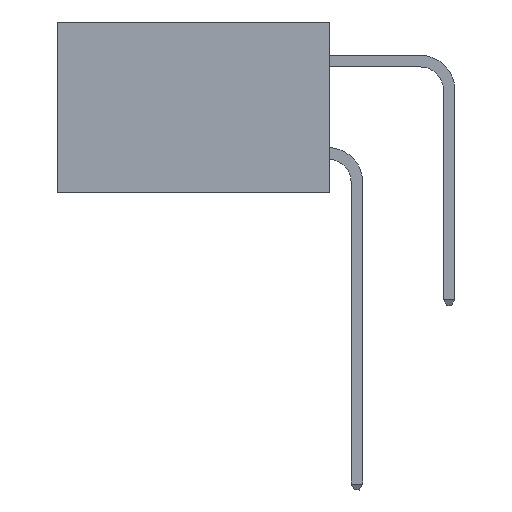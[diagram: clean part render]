
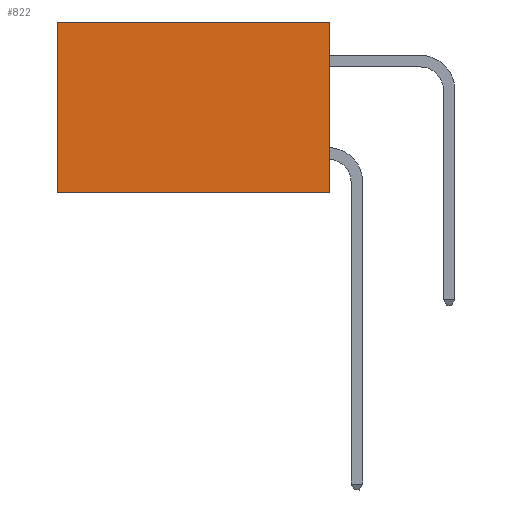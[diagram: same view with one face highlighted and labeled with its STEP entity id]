
A CAD part, left-side view. The second image highlights one B-rep face of the part: STEP entity #822.
In plain terms, the highlighted planar face has unit normal (-1, 0, 0).
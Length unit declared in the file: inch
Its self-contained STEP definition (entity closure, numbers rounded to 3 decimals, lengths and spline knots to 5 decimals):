
#822 = ADVANCED_FACE ( 'NONE', ( #1103 ), #14739, .F. ) ;
#1103 = FACE_OUTER_BOUND ( 'NONE', #1572, .T. ) ;
#1252 = VECTOR ( 'NONE', #8957, 39.37008 ) ;
#1416 = VERTEX_POINT ( 'NONE', #15825 ) ;
#1572 = EDGE_LOOP ( 'NONE', ( #16491, #4347, #13885, #8260 ) ) ;
#1595 = LINE ( 'NONE', #6151, #8107 ) ;
#1666 = LINE ( 'NONE', #16135, #8178 ) ;
#1906 = VERTEX_POINT ( 'NONE', #15460 ) ;
#2761 = VERTEX_POINT ( 'NONE', #10649 ) ;
#3179 = EDGE_CURVE ( 'NONE', #1906, #5717, #1595, .T. ) ;
#4163 = DIRECTION ( 'NONE',  ( 0., 0., -1. ) ) ;
#4347 = ORIENTED_EDGE ( 'NONE', *, *, #11721, .F. ) ;
#5587 = EDGE_CURVE ( 'NONE', #1416, #2761, #9449, .T. ) ;
#5667 = CARTESIAN_POINT ( 'NONE',  ( 0.277, 0., -0.37 ) ) ;
#5717 = VERTEX_POINT ( 'NONE', #13313 ) ;
#5975 = VECTOR ( 'NONE', #13155, 39.37008 ) ;
#6151 = CARTESIAN_POINT ( 'NONE',  ( 0.277, 0.59, -0.37 ) ) ;
#7239 = DIRECTION ( 'NONE',  ( 0., 1., 0. ) ) ;
#7612 = AXIS2_PLACEMENT_3D ( 'NONE', #5667, #14721, #14703 ) ;
#8107 = VECTOR ( 'NONE', #4163, 39.37008 ) ;
#8178 = VECTOR ( 'NONE', #7239, 39.37008 ) ;
#8260 = ORIENTED_EDGE ( 'NONE', *, *, #15944, .T. ) ;
#8957 = DIRECTION ( 'NONE',  ( 0., 1., 0. ) ) ;
#9449 = LINE ( 'NONE', #13101, #5975 ) ;
#10649 = CARTESIAN_POINT ( 'NONE',  ( 0.277, 0., -0.37 ) ) ;
#10797 = LINE ( 'NONE', #16573, #1252 ) ;
#11721 = EDGE_CURVE ( 'NONE', #2761, #5717, #1666, .T. ) ;
#13101 = CARTESIAN_POINT ( 'NONE',  ( 0.277, 0., -0.37 ) ) ;
#13155 = DIRECTION ( 'NONE',  ( 0., 0., -1. ) ) ;
#13313 = CARTESIAN_POINT ( 'NONE',  ( 0.277, 0.59, -0.37 ) ) ;
#13885 = ORIENTED_EDGE ( 'NONE', *, *, #5587, .F. ) ;
#14703 = DIRECTION ( 'NONE',  ( 0., 0., -1. ) ) ;
#14721 = DIRECTION ( 'NONE',  ( 1., 0., 0. ) ) ;
#14739 = PLANE ( 'NONE',  #7612 ) ;
#15460 = CARTESIAN_POINT ( 'NONE',  ( 0.277, 0.59, 0. ) ) ;
#15825 = CARTESIAN_POINT ( 'NONE',  ( 0.277, 0., 0. ) ) ;
#15944 = EDGE_CURVE ( 'NONE', #1416, #1906, #10797, .T. ) ;
#16135 = CARTESIAN_POINT ( 'NONE',  ( 0.277, 0., -0.37 ) ) ;
#16491 = ORIENTED_EDGE ( 'NONE', *, *, #3179, .T. ) ;
#16573 = CARTESIAN_POINT ( 'NONE',  ( 0.277, 0., 0. ) ) ;
